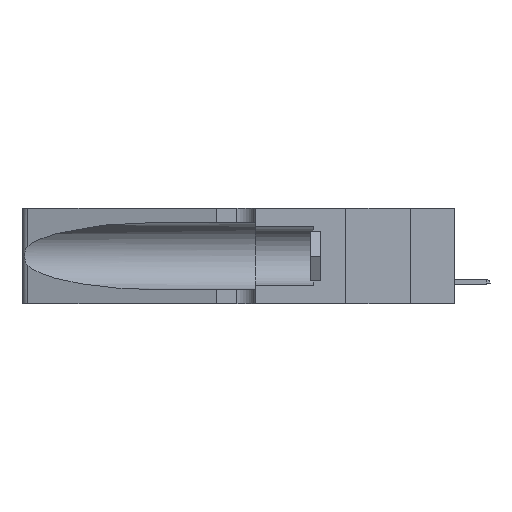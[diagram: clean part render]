
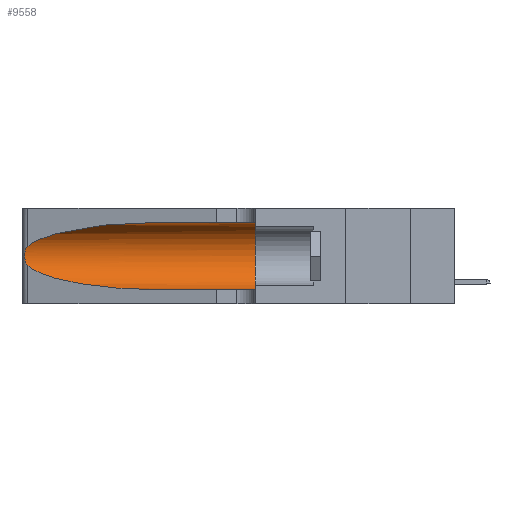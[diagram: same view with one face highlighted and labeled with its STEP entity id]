
A CAD part, left-side view. The second image highlights one B-rep face of the part: STEP entity #9558.
In plain terms, the highlighted cylindrical face has radius 3.308 mm (diameter 6.617 mm), a partial arc.
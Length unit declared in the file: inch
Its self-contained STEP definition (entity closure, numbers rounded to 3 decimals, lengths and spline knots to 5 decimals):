
#175 = VERTEX_POINT ( 'NONE', #11285 ) ;
#770 = AXIS2_PLACEMENT_3D ( 'NONE', #21600, #15958, #5727 ) ;
#1032 = CARTESIAN_POINT ( 'NONE',  ( 0.26017, 1.23833, 0.17102 ) ) ;
#1078 = CARTESIAN_POINT ( 'NONE',  ( 0.25487, 1.22718, 0.22369 ) ) ;
#1250 = CARTESIAN_POINT ( 'NONE',  ( 0.25555, 1.22993, 0.14849 ) ) ;
#1292 = CARTESIAN_POINT ( 'NONE',  ( 0.18966, 0.96281, 0.31525 ) ) ;
#2310 = VERTEX_POINT ( 'NONE', #12339 ) ;
#2847 = CARTESIAN_POINT ( 'NONE',  ( 0.25856, 1.23593, 0.16098 ) ) ;
#3045 = EDGE_CURVE ( 'NONE', #3059, #175, #3050, .T. ) ;
#3050 = LINE ( 'NONE', #15689, #8396 ) ;
#3059 = VERTEX_POINT ( 'NONE', #4785 ) ;
#3063 = CARTESIAN_POINT ( 'NONE',  ( 0.26018, 1.23835, 0.19895 ) ) ;
#3264 = ORIENTED_EDGE ( 'NONE', *, *, #13795, .T. ) ;
#4164 =( BOUNDED_CURVE ( )  B_SPLINE_CURVE ( 3, ( #11893, #7018, #4807, #15365 ),
 .UNSPECIFIED., .F., .T. ) 
 B_SPLINE_CURVE_WITH_KNOTS ( ( 4, 4 ),
 ( 3.44316, 4.71239 ),
 .UNSPECIFIED. ) 
 CURVE ( )  GEOMETRIC_REPRESENTATION_ITEM ( )  RATIONAL_B_SPLINE_CURVE ( ( 1., 0.87, 0.87, 1. ) ) 
 REPRESENTATION_ITEM ( '' )  );
#4591 = LINE ( 'NONE', #6330, #4851 ) ;
#4704 = CARTESIAN_POINT ( 'NONE',  ( 0.25555, 1.22994, 0.2215 ) ) ;
#4785 = CARTESIAN_POINT ( 'NONE',  ( 0.1305, 0.72297, 0.05475 ) ) ;
#4807 = CARTESIAN_POINT ( 'NONE',  ( 0.18966, 0.96281, 0.05475 ) ) ;
#4851 = VECTOR ( 'NONE', #9943, 39.37008 ) ;
#5034 = EDGE_CURVE ( 'NONE', #2310, #10712, #8358, .T. ) ;
#5063 = ORIENTED_EDGE ( 'NONE', *, *, #13896, .F. ) ;
#5727 = DIRECTION ( 'NONE',  ( 0., 0., 1. ) ) ;
#5823 = AXIS2_PLACEMENT_3D ( 'NONE', #17872, #16138, #7325 ) ;
#6327 = CARTESIAN_POINT ( 'NONE',  ( 0.25487, 1.22718, 0.14631 ) ) ;
#6330 = CARTESIAN_POINT ( 'NONE',  ( 0.1305, 1.61858, 0.31525 ) ) ;
#7018 = CARTESIAN_POINT ( 'NONE',  ( 0.2373, 1.15595, 0.08982 ) ) ;
#7148 = CARTESIAN_POINT ( 'NONE',  ( 0.25487, 1.22718, 0.14631 ) ) ;
#7200 = VERTEX_POINT ( 'NONE', #20054 ) ;
#7325 = DIRECTION ( 'NONE',  ( 0., 0., -1. ) ) ;
#8358 =( BOUNDED_CURVE ( )  B_SPLINE_CURVE ( 3, ( #9758, #1292, #11496, #1078 ),
 .UNSPECIFIED., .F., .T. ) 
 B_SPLINE_CURVE_WITH_KNOTS ( ( 4, 4 ),
 ( 1.5708, 2.84003 ),
 .UNSPECIFIED. ) 
 CURVE ( )  GEOMETRIC_REPRESENTATION_ITEM ( )  RATIONAL_B_SPLINE_CURVE ( ( 1., 0.87, 0.87, 1. ) ) 
 REPRESENTATION_ITEM ( '' )  );
#8396 = VECTOR ( 'NONE', #22741, 39.37008 ) ;
#9080 = VERTEX_POINT ( 'NONE', #7148 ) ;
#9558 = ADVANCED_FACE ( 'NONE', ( #10816 ), #12775, .F. ) ;
#9758 = CARTESIAN_POINT ( 'NONE',  ( 0.1305, 0.72297, 0.31525 ) ) ;
#9822 = CARTESIAN_POINT ( 'NONE',  ( 0.25787, 1.23484, 0.2124 ) ) ;
#9941 = CARTESIAN_POINT ( 'NONE',  ( 0.26075, 1.23896, 0.19203 ) ) ;
#9943 = DIRECTION ( 'NONE',  ( 0., -1., 0. ) ) ;
#10712 = VERTEX_POINT ( 'NONE', #19152 ) ;
#10816 = FACE_OUTER_BOUND ( 'NONE', #22673, .T. ) ;
#11285 = CARTESIAN_POINT ( 'NONE',  ( 0.1305, 0.35, 0.05475 ) ) ;
#11496 = CARTESIAN_POINT ( 'NONE',  ( 0.2373, 1.15595, 0.28018 ) ) ;
#11893 = CARTESIAN_POINT ( 'NONE',  ( 0.25487, 1.22718, 0.14631 ) ) ;
#12339 = CARTESIAN_POINT ( 'NONE',  ( 0.1305, 0.72297, 0.31525 ) ) ;
#12775 = CYLINDRICAL_SURFACE ( 'NONE', #5823, 0.13025 ) ;
#13523 = CARTESIAN_POINT ( 'NONE',  ( 0.26075, 1.23896, 0.178 ) ) ;
#13749 = CARTESIAN_POINT ( 'NONE',  ( 0.25854, 1.2359, 0.20912 ) ) ;
#13795 = EDGE_CURVE ( 'NONE', #9080, #3059, #4164, .T. ) ;
#13896 = EDGE_CURVE ( 'NONE', #7200, #175, #15182, .T. ) ;
#14213 = ORIENTED_EDGE ( 'NONE', *, *, #3045, .T. ) ;
#14891 = ORIENTED_EDGE ( 'NONE', *, *, #5034, .T. ) ;
#15182 = CIRCLE ( 'NONE', #770, 0.13025 ) ;
#15365 = CARTESIAN_POINT ( 'NONE',  ( 0.1305, 0.72297, 0.05475 ) ) ;
#15689 = CARTESIAN_POINT ( 'NONE',  ( 0.1305, 1.61858, 0.05475 ) ) ;
#15958 = DIRECTION ( 'NONE',  ( 0., 1., 0. ) ) ;
#15967 = EDGE_CURVE ( 'NONE', #2310, #7200, #4591, .T. ) ;
#16138 = DIRECTION ( 'NONE',  ( 0., -1., 0. ) ) ;
#16989 = CARTESIAN_POINT ( 'NONE',  ( 0.25789, 1.23486, 0.15765 ) ) ;
#17116 = CARTESIAN_POINT ( 'NONE',  ( 0.25487, 1.22718, 0.22369 ) ) ;
#17872 = CARTESIAN_POINT ( 'NONE',  ( 0.1305, 1.61858, 0.185 ) ) ;
#18326 = B_SPLINE_CURVE_WITH_KNOTS ( 'NONE', 3,
 ( #17116, #4704, #20410, #9822, #13749, #3063, #9941, #13523, #1032, #2847, #16989, #20767, #1250, #6327 ),
 .UNSPECIFIED., .F., .F.,
 ( 4, 2, 2, 2, 2, 2, 4 ),
 ( 0., 0.00027, 0.00053, 0.00107, 0.0016, 0.00187, 0.00214 ),
 .UNSPECIFIED. ) ;
#18621 = EDGE_CURVE ( 'NONE', #10712, #9080, #18326, .T. ) ;
#19053 = ORIENTED_EDGE ( 'NONE', *, *, #18621, .T. ) ;
#19152 = CARTESIAN_POINT ( 'NONE',  ( 0.25487, 1.22718, 0.22369 ) ) ;
#20054 = CARTESIAN_POINT ( 'NONE',  ( 0.1305, 0.35, 0.31525 ) ) ;
#20410 = CARTESIAN_POINT ( 'NONE',  ( 0.25639, 1.23184, 0.21858 ) ) ;
#20574 = ORIENTED_EDGE ( 'NONE', *, *, #15967, .F. ) ;
#20767 = CARTESIAN_POINT ( 'NONE',  ( 0.25639, 1.23186, 0.15144 ) ) ;
#21600 = CARTESIAN_POINT ( 'NONE',  ( 0.1305, 0.35, 0.185 ) ) ;
#22673 = EDGE_LOOP ( 'NONE', ( #14891, #19053, #3264, #14213, #5063, #20574 ) ) ;
#22741 = DIRECTION ( 'NONE',  ( 0., -1., 0. ) ) ;
